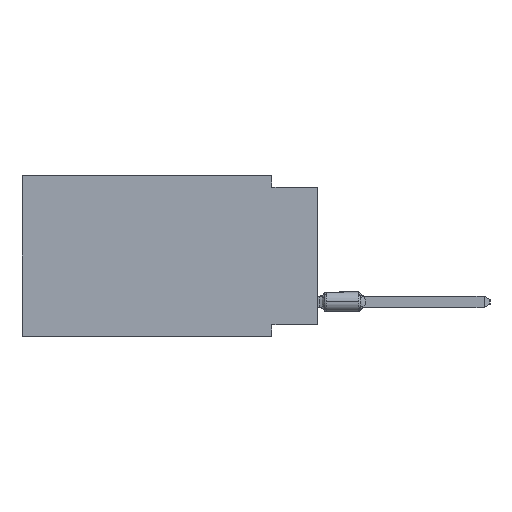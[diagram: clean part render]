
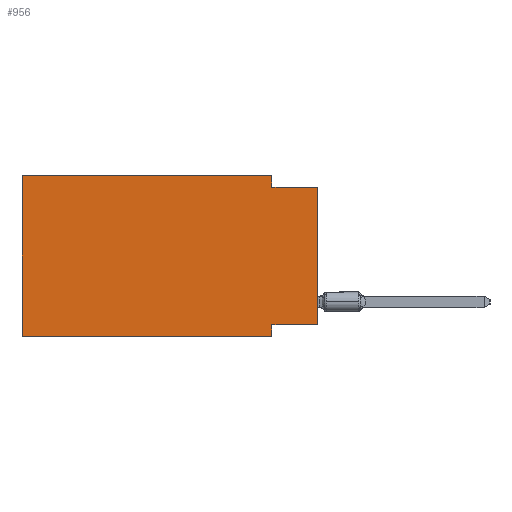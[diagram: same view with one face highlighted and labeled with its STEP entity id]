
A CAD part, left-side view. The second image highlights one B-rep face of the part: STEP entity #956.
In plain terms, the highlighted planar face has unit normal (-1, 0, 0).
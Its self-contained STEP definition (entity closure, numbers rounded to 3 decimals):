
#956 = ADVANCED_FACE ( 'NONE', ( #40147 ), #4175, .F. ) ;
#1061 = CARTESIAN_POINT ( 'NONE',  ( 0., 16.383, -8.89 ) ) ;
#1378 = CARTESIAN_POINT ( 'NONE',  ( 0., 2.54, 0. ) ) ;
#1433 = VERTEX_POINT ( 'NONE', #1704 ) ;
#1704 = CARTESIAN_POINT ( 'NONE',  ( 0., 2.54, -8.89 ) ) ;
#1958 = CARTESIAN_POINT ( 'NONE',  ( 0., 16.383, 0. ) ) ;
#4175 = PLANE ( 'NONE',  #40259 ) ;
#4558 = DIRECTION ( 'NONE',  ( 0., -1., 0. ) ) ;
#4695 = CARTESIAN_POINT ( 'NONE',  ( 0., 2.54, 0. ) ) ;
#4843 = LINE ( 'NONE', #27606, #6417 ) ;
#5431 = LINE ( 'NONE', #1958, #7707 ) ;
#6417 = VECTOR ( 'NONE', #14592, 1000. ) ;
#6492 = LINE ( 'NONE', #12316, #35480 ) ;
#6994 = LINE ( 'NONE', #19992, #14496 ) ;
#7523 = VECTOR ( 'NONE', #4558, 1000. ) ;
#7707 = VECTOR ( 'NONE', #18032, 1000. ) ;
#7767 = ORIENTED_EDGE ( 'NONE', *, *, #12947, .T. ) ;
#7818 = LINE ( 'NONE', #21036, #7523 ) ;
#8503 = VERTEX_POINT ( 'NONE', #31297 ) ;
#8741 = LINE ( 'NONE', #1378, #37755 ) ;
#10214 = DIRECTION ( 'NONE',  ( 0., 0., 1. ) ) ;
#10896 = VERTEX_POINT ( 'NONE', #4695 ) ;
#12255 = ORIENTED_EDGE ( 'NONE', *, *, #30487, .F. ) ;
#12316 = CARTESIAN_POINT ( 'NONE',  ( 0., 0., -8.255 ) ) ;
#12342 = DIRECTION ( 'NONE',  ( 0., -1., 0. ) ) ;
#12947 = EDGE_CURVE ( 'NONE', #27357, #18294, #6994, .T. ) ;
#13048 = DIRECTION ( 'NONE',  ( 0., 0., -1. ) ) ;
#14270 = EDGE_CURVE ( 'NONE', #23174, #1433, #35100, .T. ) ;
#14496 = VECTOR ( 'NONE', #10214, 1000. ) ;
#14592 = DIRECTION ( 'NONE',  ( 0., -1., 0. ) ) ;
#15544 = ORIENTED_EDGE ( 'NONE', *, *, #33587, .F. ) ;
#15816 = EDGE_CURVE ( 'NONE', #23174, #28123, #5431, .T. ) ;
#16594 = CARTESIAN_POINT ( 'NONE',  ( 0., 16.383, 0. ) ) ;
#17297 = VERTEX_POINT ( 'NONE', #27114 ) ;
#17403 = DIRECTION ( 'NONE',  ( 1., 0., 0. ) ) ;
#17577 = EDGE_CURVE ( 'NONE', #27357, #17297, #6492, .T. ) ;
#18032 = DIRECTION ( 'NONE',  ( 0., 0., 1. ) ) ;
#18294 = VERTEX_POINT ( 'NONE', #19108 ) ;
#18652 = VECTOR ( 'NONE', #12342, 1000. ) ;
#19108 = CARTESIAN_POINT ( 'NONE',  ( 0., 0., -0.635 ) ) ;
#19517 = ORIENTED_EDGE ( 'NONE', *, *, #14270, .T. ) ;
#19992 = CARTESIAN_POINT ( 'NONE',  ( 0., 0., 0. ) ) ;
#21036 = CARTESIAN_POINT ( 'NONE',  ( 0., 0., -0.635 ) ) ;
#21246 = ORIENTED_EDGE ( 'NONE', *, *, #36572, .F. ) ;
#21692 = CARTESIAN_POINT ( 'NONE',  ( 0., 16.383, -8.89 ) ) ;
#23174 = VERTEX_POINT ( 'NONE', #1061 ) ;
#24076 = EDGE_CURVE ( 'NONE', #28123, #10896, #4843, .T. ) ;
#25634 = CARTESIAN_POINT ( 'NONE',  ( 0., 2.54, -8.89 ) ) ;
#26461 = CARTESIAN_POINT ( 'NONE',  ( 0., 0., -8.255 ) ) ;
#27114 = CARTESIAN_POINT ( 'NONE',  ( 0., 2.54, -8.255 ) ) ;
#27357 = VERTEX_POINT ( 'NONE', #26461 ) ;
#27606 = CARTESIAN_POINT ( 'NONE',  ( 0., 16.383, 0. ) ) ;
#28026 = EDGE_LOOP ( 'NONE', ( #7767, #15544, #12255, #41502, #39840, #19517, #21246, #34772 ) ) ;
#28123 = VERTEX_POINT ( 'NONE', #16594 ) ;
#30487 = EDGE_CURVE ( 'NONE', #10896, #8503, #8741, .T. ) ;
#30628 = DIRECTION ( 'NONE',  ( 0., 0., -1. ) ) ;
#31297 = CARTESIAN_POINT ( 'NONE',  ( 0., 2.54, -0.635 ) ) ;
#33587 = EDGE_CURVE ( 'NONE', #8503, #18294, #7818, .T. ) ;
#34754 = DIRECTION ( 'NONE',  ( 0., 0., -1. ) ) ;
#34772 = ORIENTED_EDGE ( 'NONE', *, *, #17577, .F. ) ;
#35100 = LINE ( 'NONE', #21692, #18652 ) ;
#35480 = VECTOR ( 'NONE', #42656, 1000. ) ;
#36572 = EDGE_CURVE ( 'NONE', #17297, #1433, #42514, .T. ) ;
#37755 = VECTOR ( 'NONE', #34754, 1000. ) ;
#39840 = ORIENTED_EDGE ( 'NONE', *, *, #15816, .F. ) ;
#40147 = FACE_OUTER_BOUND ( 'NONE', #28026, .T. ) ;
#40259 = AXIS2_PLACEMENT_3D ( 'NONE', #40361, #17403, #30628 ) ;
#40361 = CARTESIAN_POINT ( 'NONE',  ( 0., 16.383, 0. ) ) ;
#41187 = VECTOR ( 'NONE', #13048, 1000. ) ;
#41502 = ORIENTED_EDGE ( 'NONE', *, *, #24076, .F. ) ;
#42514 = LINE ( 'NONE', #25634, #41187 ) ;
#42656 = DIRECTION ( 'NONE',  ( 0., 1., 0. ) ) ;
